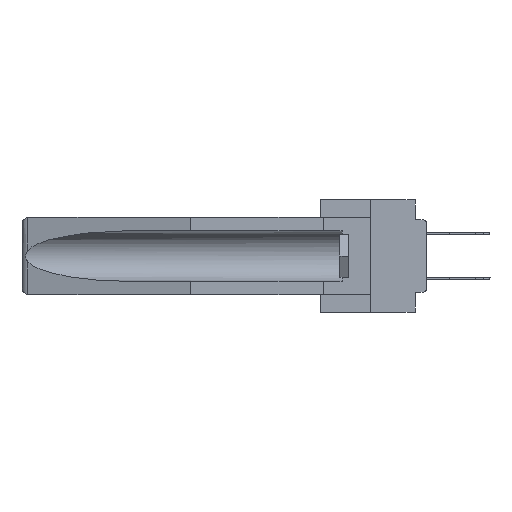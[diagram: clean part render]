
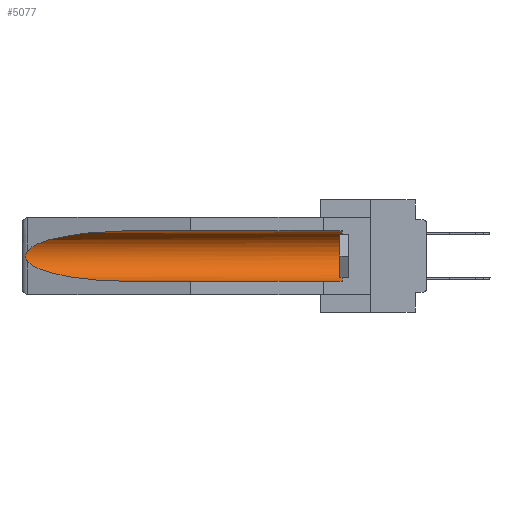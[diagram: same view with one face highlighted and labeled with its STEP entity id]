
A CAD part, left-side view. The second image highlights one B-rep face of the part: STEP entity #5077.
In plain terms, the highlighted cylindrical face has radius 2.857 mm (diameter 5.715 mm), a partial arc.
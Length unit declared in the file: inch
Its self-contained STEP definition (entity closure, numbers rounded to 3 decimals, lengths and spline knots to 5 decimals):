
#886 = VERTEX_POINT ( 'NONE', #4765 ) ;
#1161 = CARTESIAN_POINT ( 'NONE',  ( 0.21114, 1.30732, -0.284 ) ) ;
#1369 = VERTEX_POINT ( 'NONE', #8739 ) ;
#2024 = ORIENTED_EDGE ( 'NONE', *, *, #10165, .T. ) ;
#2892 = DIRECTION ( 'NONE',  ( 0., 1., 0. ) ) ;
#2905 = CARTESIAN_POINT ( 'NONE',  ( 0.26537, 1.52718, -0.14972 ) ) ;
#2944 = CARTESIAN_POINT ( 'NONE',  ( 0.21114, 1.30732, -0.059 ) ) ;
#3122 = CARTESIAN_POINT ( 'NONE',  ( 0.2675, 1.53308, -0.17534 ) ) ;
#3261 = EDGE_CURVE ( 'NONE', #886, #4492, #4705, .T. ) ;
#4388 = VECTOR ( 'NONE', #2892, 39.37008 ) ;
#4418 = VERTEX_POINT ( 'NONE', #25932 ) ;
#4492 = VERTEX_POINT ( 'NONE', #8024 ) ;
#4705 =( BOUNDED_CURVE ( )  B_SPLINE_CURVE ( 3, ( #13157, #2944, #31188, #10868 ),
 .UNSPECIFIED., .F., .F. ) 
 B_SPLINE_CURVE_WITH_KNOTS ( ( 4, 4 ),
 ( 4.71239, 6.08839 ),
 .UNSPECIFIED. ) 
 CURVE ( )  GEOMETRIC_REPRESENTATION_ITEM ( )  RATIONAL_B_SPLINE_CURVE ( ( 1., 0.848, 0.848, 1. ) ) 
 REPRESENTATION_ITEM ( '' )  );
#4765 = CARTESIAN_POINT ( 'NONE',  ( 0.155, 1.07973, -0.059 ) ) ;
#4968 = CARTESIAN_POINT ( 'NONE',  ( 0.155, 0.126, -0.059 ) ) ;
#5077 = ADVANCED_FACE ( 'NONE', ( #29162 ), #29992, .F. ) ;
#5515 = CARTESIAN_POINT ( 'NONE',  ( 0.26654, 1.53092, -0.15636 ) ) ;
#5738 = CARTESIAN_POINT ( 'NONE',  ( 0.26597, 1.52961, -0.15275 ) ) ;
#5800 = B_SPLINE_CURVE_WITH_KNOTS ( 'NONE', 3,
 ( #2905, #5738, #5515, #31372, #18670, #3122, #28860, #18457, #26366, #8472 ),
 .UNSPECIFIED., .F., .F.,
 ( 4, 2, 2, 2, 4 ),
 ( 0., 0.00029, 0.00058, 0.00087, 0.00117 ),
 .UNSPECIFIED. ) ;
#6743 = VECTOR ( 'NONE', #17965, 39.37008 ) ;
#8024 = CARTESIAN_POINT ( 'NONE',  ( 0.26537, 1.52718, -0.14972 ) ) ;
#8093 = CARTESIAN_POINT ( 'NONE',  ( 0.155, -0.30754, -0.1715 ) ) ;
#8205 = DIRECTION ( 'NONE',  ( 0., 1., 0. ) ) ;
#8292 = EDGE_CURVE ( 'NONE', #16472, #27296, #22053, .T. ) ;
#8472 = CARTESIAN_POINT ( 'NONE',  ( 0.26537, 1.52718, -0.19328 ) ) ;
#8685 = AXIS2_PLACEMENT_3D ( 'NONE', #8712, #16528, #26826 ) ;
#8712 = CARTESIAN_POINT ( 'NONE',  ( 0.155, 0.126, -0.1715 ) ) ;
#8739 = CARTESIAN_POINT ( 'NONE',  ( 0.155, 1.07973, -0.284 ) ) ;
#9034 = EDGE_CURVE ( 'NONE', #16472, #1369, #32397, .T. ) ;
#9115 = CARTESIAN_POINT ( 'NONE',  ( 0.26537, 1.52718, -0.19328 ) ) ;
#9177 = LINE ( 'NONE', #10462, #6743 ) ;
#9186 = ORIENTED_EDGE ( 'NONE', *, *, #21154, .T. ) ;
#10165 = EDGE_CURVE ( 'NONE', #27296, #886, #9177, .T. ) ;
#10462 = CARTESIAN_POINT ( 'NONE',  ( 0.155, -0.30754, -0.059 ) ) ;
#10868 = CARTESIAN_POINT ( 'NONE',  ( 0.26537, 1.52718, -0.14972 ) ) ;
#13078 = DIRECTION ( 'NONE',  ( 0., 0., 1. ) ) ;
#13157 = CARTESIAN_POINT ( 'NONE',  ( 0.155, 1.07973, -0.059 ) ) ;
#15159 = EDGE_LOOP ( 'NONE', ( #28198, #30088, #9186, #17714, #16701, #2024 ) ) ;
#16042 = CARTESIAN_POINT ( 'NONE',  ( 0.155, -0.30754, -0.284 ) ) ;
#16472 = VERTEX_POINT ( 'NONE', #25235 ) ;
#16528 = DIRECTION ( 'NONE',  ( 0., -1., 0. ) ) ;
#16701 = ORIENTED_EDGE ( 'NONE', *, *, #8292, .T. ) ;
#17714 = ORIENTED_EDGE ( 'NONE', *, *, #9034, .F. ) ;
#17965 = DIRECTION ( 'NONE',  ( 0., 1., 0. ) ) ;
#18457 = CARTESIAN_POINT ( 'NONE',  ( 0.26655, 1.53094, -0.18657 ) ) ;
#18631 = AXIS2_PLACEMENT_3D ( 'NONE', #8093, #8205, #13078 ) ;
#18670 = CARTESIAN_POINT ( 'NONE',  ( 0.2675, 1.53308, -0.16763 ) ) ;
#19871 =( BOUNDED_CURVE ( )  B_SPLINE_CURVE ( 3, ( #9115, #26895, #1161, #24647 ),
 .UNSPECIFIED., .F., .F. ) 
 B_SPLINE_CURVE_WITH_KNOTS ( ( 4, 4 ),
 ( 0.1948, 1.5708 ),
 .UNSPECIFIED. ) 
 CURVE ( )  GEOMETRIC_REPRESENTATION_ITEM ( )  RATIONAL_B_SPLINE_CURVE ( ( 1., 0.848, 0.848, 1. ) ) 
 REPRESENTATION_ITEM ( '' )  );
#21154 = EDGE_CURVE ( 'NONE', #4418, #1369, #19871, .T. ) ;
#22053 = CIRCLE ( 'NONE', #8685, 0.1125 ) ;
#23822 = EDGE_CURVE ( 'NONE', #4492, #4418, #5800, .T. ) ;
#24647 = CARTESIAN_POINT ( 'NONE',  ( 0.155, 1.07973, -0.284 ) ) ;
#25235 = CARTESIAN_POINT ( 'NONE',  ( 0.155, 0.126, -0.284 ) ) ;
#25932 = CARTESIAN_POINT ( 'NONE',  ( 0.26537, 1.52718, -0.19328 ) ) ;
#26366 = CARTESIAN_POINT ( 'NONE',  ( 0.26597, 1.5296, -0.19026 ) ) ;
#26826 = DIRECTION ( 'NONE',  ( 0., 0., 1. ) ) ;
#26895 = CARTESIAN_POINT ( 'NONE',  ( 0.25451, 1.48313, -0.24835 ) ) ;
#27296 = VERTEX_POINT ( 'NONE', #4968 ) ;
#28198 = ORIENTED_EDGE ( 'NONE', *, *, #3261, .T. ) ;
#28860 = CARTESIAN_POINT ( 'NONE',  ( 0.2673, 1.53269, -0.17917 ) ) ;
#29162 = FACE_OUTER_BOUND ( 'NONE', #15159, .T. ) ;
#29992 = CYLINDRICAL_SURFACE ( 'NONE', #18631, 0.1125 ) ;
#30088 = ORIENTED_EDGE ( 'NONE', *, *, #23822, .T. ) ;
#31188 = CARTESIAN_POINT ( 'NONE',  ( 0.25451, 1.48313, -0.09465 ) ) ;
#31372 = CARTESIAN_POINT ( 'NONE',  ( 0.2673, 1.5327, -0.16383 ) ) ;
#32397 = LINE ( 'NONE', #16042, #4388 ) ;
